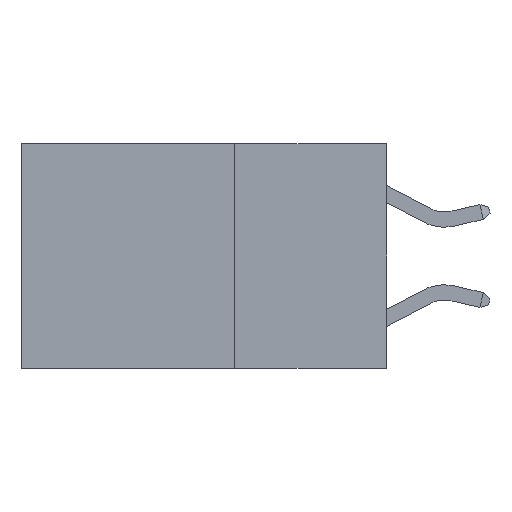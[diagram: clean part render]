
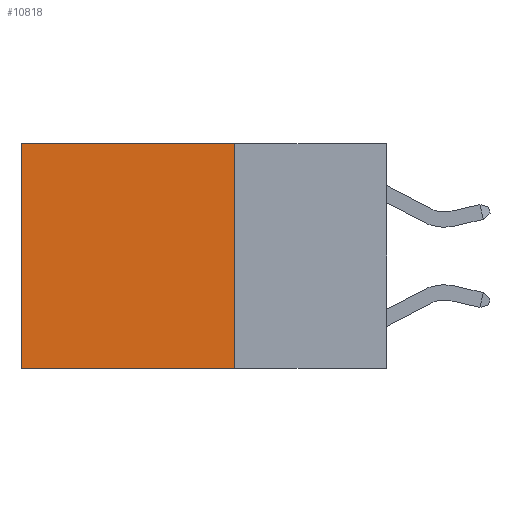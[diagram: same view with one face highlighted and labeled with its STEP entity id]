
A CAD part, left-side view. The second image highlights one B-rep face of the part: STEP entity #10818.
In plain terms, the highlighted planar face has unit normal (-1, 0, 0).
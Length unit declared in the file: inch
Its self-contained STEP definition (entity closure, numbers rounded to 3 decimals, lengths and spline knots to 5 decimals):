
#581 = CARTESIAN_POINT ( 'NONE',  ( 0.2625, 0.6, 0. ) ) ;
#678 = CARTESIAN_POINT ( 'NONE',  ( 0.2625, 0.25, 0. ) ) ;
#1067 = CARTESIAN_POINT ( 'NONE',  ( 0.2625, 0.25, -0.37 ) ) ;
#1419 = DIRECTION ( 'NONE',  ( 0., 1., 0. ) ) ;
#1550 = VERTEX_POINT ( 'NONE', #3906 ) ;
#1676 = DIRECTION ( 'NONE',  ( 1., 0., 0. ) ) ;
#1747 = VERTEX_POINT ( 'NONE', #11333 ) ;
#1966 = EDGE_CURVE ( 'NONE', #8015, #1747, #3738, .T. ) ;
#2390 = VERTEX_POINT ( 'NONE', #3008 ) ;
#3008 = CARTESIAN_POINT ( 'NONE',  ( 0.2625, 0.6, 0. ) ) ;
#3179 = EDGE_LOOP ( 'NONE', ( #7330, #4075, #3486, #6603 ) ) ;
#3360 = CARTESIAN_POINT ( 'NONE',  ( 0.2625, 0.25, -0.37 ) ) ;
#3436 = EDGE_CURVE ( 'NONE', #2390, #1747, #11326, .T. ) ;
#3486 = ORIENTED_EDGE ( 'NONE', *, *, #7748, .F. ) ;
#3640 = FACE_OUTER_BOUND ( 'NONE', #3179, .T. ) ;
#3738 = LINE ( 'NONE', #3360, #12050 ) ;
#3906 = CARTESIAN_POINT ( 'NONE',  ( 0.2625, 0.25, 0. ) ) ;
#4075 = ORIENTED_EDGE ( 'NONE', *, *, #1966, .F. ) ;
#4889 = DIRECTION ( 'NONE',  ( 0., 0., -1. ) ) ;
#5171 = LINE ( 'NONE', #7422, #10463 ) ;
#6284 = DIRECTION ( 'NONE',  ( 0., 1., 0. ) ) ;
#6603 = ORIENTED_EDGE ( 'NONE', *, *, #12506, .T. ) ;
#6679 = VECTOR ( 'NONE', #4889, 39.37008 ) ;
#6704 = PLANE ( 'NONE',  #10994 ) ;
#7330 = ORIENTED_EDGE ( 'NONE', *, *, #3436, .T. ) ;
#7422 = CARTESIAN_POINT ( 'NONE',  ( 0.2625, 0.25, 0. ) ) ;
#7748 = EDGE_CURVE ( 'NONE', #1550, #8015, #9952, .T. ) ;
#8015 = VERTEX_POINT ( 'NONE', #1067 ) ;
#8323 = VECTOR ( 'NONE', #8615, 39.37008 ) ;
#8615 = DIRECTION ( 'NONE',  ( 0., 0., -1. ) ) ;
#8715 = DIRECTION ( 'NONE',  ( 0., 0., -1. ) ) ;
#9887 = CARTESIAN_POINT ( 'NONE',  ( 0.2625, 0.25, 0. ) ) ;
#9952 = LINE ( 'NONE', #9887, #6679 ) ;
#10463 = VECTOR ( 'NONE', #1419, 39.37008 ) ;
#10818 = ADVANCED_FACE ( 'NONE', ( #3640 ), #6704, .F. ) ;
#10994 = AXIS2_PLACEMENT_3D ( 'NONE', #678, #1676, #8715 ) ;
#11326 = LINE ( 'NONE', #581, #8323 ) ;
#11333 = CARTESIAN_POINT ( 'NONE',  ( 0.2625, 0.6, -0.37 ) ) ;
#12050 = VECTOR ( 'NONE', #6284, 39.37008 ) ;
#12506 = EDGE_CURVE ( 'NONE', #1550, #2390, #5171, .T. ) ;
